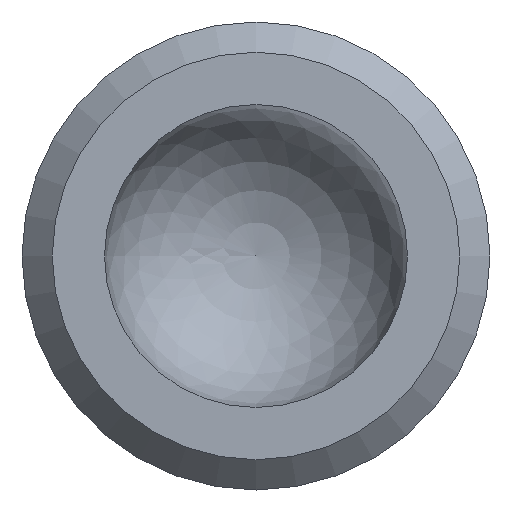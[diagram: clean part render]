
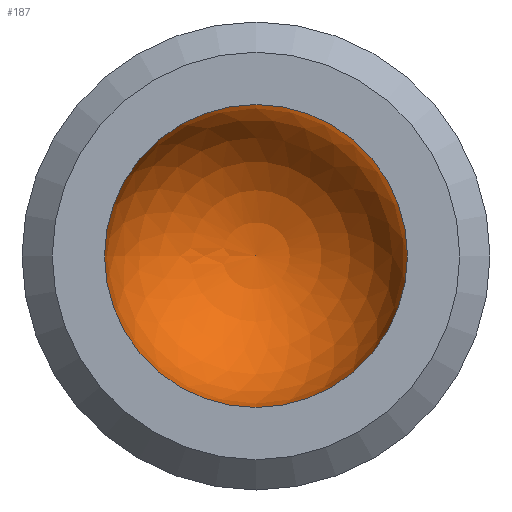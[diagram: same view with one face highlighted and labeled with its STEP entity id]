
A CAD part, left-side view. The second image highlights one B-rep face of the part: STEP entity #187.
In plain terms, the highlighted spherical face has radius 1.27 mm.
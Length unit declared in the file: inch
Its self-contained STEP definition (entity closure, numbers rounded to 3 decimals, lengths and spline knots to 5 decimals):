
#19=SPHERICAL_SURFACE('',#223,0.05);
#35=FACE_OUTER_BOUND('',#50,.T.);
#50=EDGE_LOOP('',(#151,#152,#153));
#74=CIRCLE('',#218,0.05);
#77=CIRCLE('',#224,0.05);
#93=VERTEX_POINT('',#332);
#96=VERTEX_POINT('',#342);
#112=EDGE_CURVE('',#93,#93,#74,.T.);
#116=EDGE_CURVE('',#93,#96,#77,.T.);
#151=ORIENTED_EDGE('',*,*,#112,.F.);
#152=ORIENTED_EDGE('',*,*,#116,.T.);
#153=ORIENTED_EDGE('',*,*,#116,.F.);
#187=ADVANCED_FACE('',(#35),#19,.F.);
#218=AXIS2_PLACEMENT_3D('',#333,#266,#267);
#223=AXIS2_PLACEMENT_3D('',#341,#277,#278);
#224=AXIS2_PLACEMENT_3D('',#343,#279,#280);
#266=DIRECTION('center_axis',(1.,0.,0.));
#267=DIRECTION('ref_axis',(0.,0.,-1.));
#277=DIRECTION('center_axis',(1.,0.,0.));
#278=DIRECTION('ref_axis',(0.,-1.,0.));
#279=DIRECTION('center_axis',(0.,0.,-1.));
#280=DIRECTION('ref_axis',(0.,1.,0.));
#332=CARTESIAN_POINT('',(0.,0.05,0.));
#333=CARTESIAN_POINT('Origin',(0.,0.,0.));
#341=CARTESIAN_POINT('Origin',(0.,0.,0.));
#342=CARTESIAN_POINT('',(0.05,0.,0.));
#343=CARTESIAN_POINT('Origin',(0.,0.,0.));
